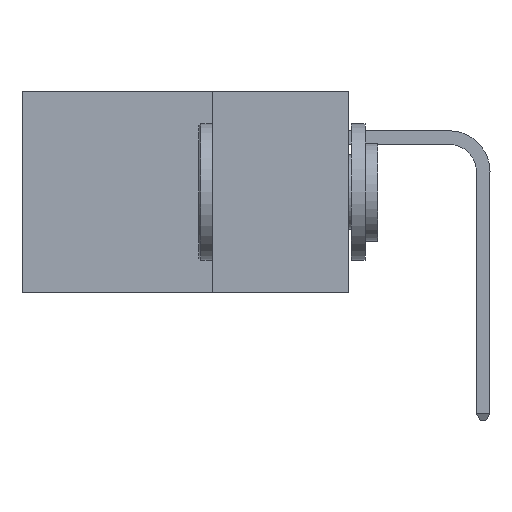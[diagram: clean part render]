
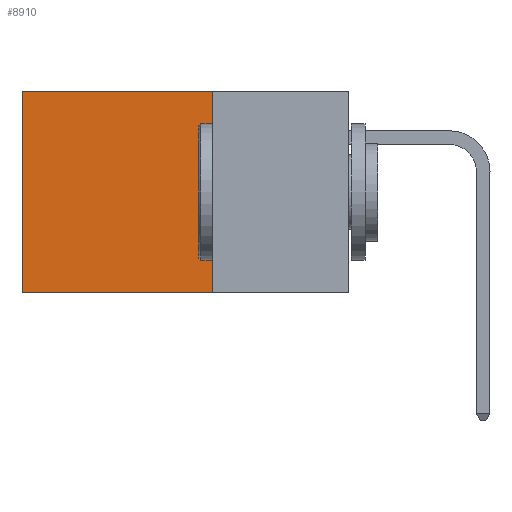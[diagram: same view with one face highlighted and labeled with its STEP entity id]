
A CAD part, left-side view. The second image highlights one B-rep face of the part: STEP entity #8910.
In plain terms, the highlighted planar face has unit normal (-1, 0, 0).
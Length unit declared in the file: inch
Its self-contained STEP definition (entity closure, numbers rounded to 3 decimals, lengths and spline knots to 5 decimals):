
#19 = FACE_OUTER_BOUND ( 'NONE', #13538, .T. ) ;
#1993 = EDGE_CURVE ( 'NONE', #30805, #35247, #3307, .T. ) ;
#2467 = CARTESIAN_POINT ( 'NONE',  ( 0.2875, 0.25, 0. ) ) ;
#2852 = CARTESIAN_POINT ( 'NONE',  ( 0.2875, 0.6, 0. ) ) ;
#3307 = LINE ( 'NONE', #16010, #24204 ) ;
#4282 = ORIENTED_EDGE ( 'NONE', *, *, #1993, .F. ) ;
#7800 = VECTOR ( 'NONE', #25524, 39.37008 ) ;
#8424 = CARTESIAN_POINT ( 'NONE',  ( 0.2875, 0.25, 0. ) ) ;
#8508 = EDGE_CURVE ( 'NONE', #12082, #32802, #17217, .T. ) ;
#8910 = ADVANCED_FACE ( 'NONE', ( #19 ), #30315, .F. ) ;
#9061 = VECTOR ( 'NONE', #28872, 39.37008 ) ;
#11444 = ORIENTED_EDGE ( 'NONE', *, *, #8508, .T. ) ;
#12082 = VERTEX_POINT ( 'NONE', #2467 ) ;
#12441 = DIRECTION ( 'NONE',  ( 0., 0., -1. ) ) ;
#12805 = EDGE_CURVE ( 'NONE', #12082, #30805, #31195, .T. ) ;
#13538 = EDGE_LOOP ( 'NONE', ( #28416, #4282, #32318, #11444 ) ) ;
#14758 = CARTESIAN_POINT ( 'NONE',  ( 0.2875, 0.6, 0. ) ) ;
#16010 = CARTESIAN_POINT ( 'NONE',  ( 0.2875, 0.25, -0.37 ) ) ;
#16244 = CARTESIAN_POINT ( 'NONE',  ( 0.2875, 0.25, 0. ) ) ;
#16569 = AXIS2_PLACEMENT_3D ( 'NONE', #16244, #35954, #19104 ) ;
#16570 = DIRECTION ( 'NONE',  ( 0., 1., 0. ) ) ;
#17217 = LINE ( 'NONE', #8424, #7800 ) ;
#19104 = DIRECTION ( 'NONE',  ( 0., 0., -1. ) ) ;
#21879 = CARTESIAN_POINT ( 'NONE',  ( 0.2875, 0.6, -0.37 ) ) ;
#24204 = VECTOR ( 'NONE', #16570, 39.37008 ) ;
#25524 = DIRECTION ( 'NONE',  ( 0., 1., 0. ) ) ;
#26522 = CARTESIAN_POINT ( 'NONE',  ( 0.2875, 0.25, 0. ) ) ;
#28416 = ORIENTED_EDGE ( 'NONE', *, *, #30852, .T. ) ;
#28872 = DIRECTION ( 'NONE',  ( 0., 0., -1. ) ) ;
#30315 = PLANE ( 'NONE',  #16569 ) ;
#30780 = LINE ( 'NONE', #14758, #9061 ) ;
#30805 = VERTEX_POINT ( 'NONE', #34282 ) ;
#30852 = EDGE_CURVE ( 'NONE', #32802, #35247, #30780, .T. ) ;
#31195 = LINE ( 'NONE', #26522, #36848 ) ;
#32318 = ORIENTED_EDGE ( 'NONE', *, *, #12805, .F. ) ;
#32802 = VERTEX_POINT ( 'NONE', #2852 ) ;
#34282 = CARTESIAN_POINT ( 'NONE',  ( 0.2875, 0.25, -0.37 ) ) ;
#35247 = VERTEX_POINT ( 'NONE', #21879 ) ;
#35954 = DIRECTION ( 'NONE',  ( 1., 0., 0. ) ) ;
#36848 = VECTOR ( 'NONE', #12441, 39.37008 ) ;
